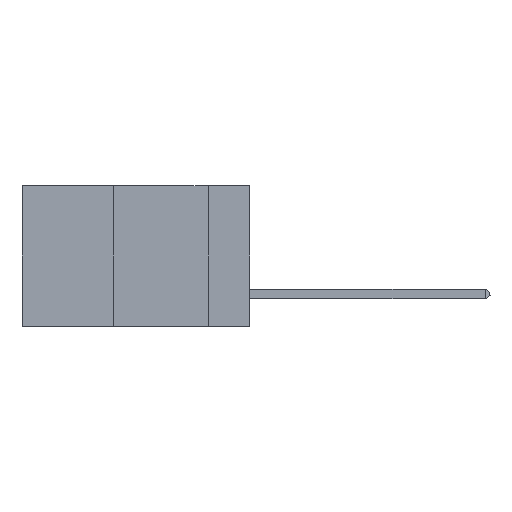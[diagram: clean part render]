
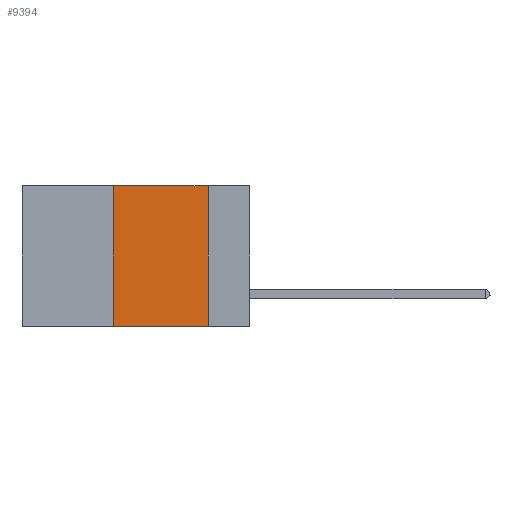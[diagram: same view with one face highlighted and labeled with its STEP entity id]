
A CAD part, left-side view. The second image highlights one B-rep face of the part: STEP entity #9394.
In plain terms, the highlighted planar face has unit normal (-1, 0, 0).
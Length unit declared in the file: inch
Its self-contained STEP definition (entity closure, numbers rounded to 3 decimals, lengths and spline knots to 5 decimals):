
#344 = VECTOR ( 'NONE', #7917, 39.37008 ) ;
#497 = DIRECTION ( 'NONE',  ( 0., 0., -1. ) ) ;
#654 = PLANE ( 'NONE',  #12254 ) ;
#928 = EDGE_CURVE ( 'NONE', #20056, #16907, #2650, .T. ) ;
#1216 = CARTESIAN_POINT ( 'NONE',  ( 0., 0.11, 0. ) ) ;
#1509 = DIRECTION ( 'NONE',  ( 0., -1., 0. ) ) ;
#1728 = EDGE_LOOP ( 'NONE', ( #21644, #12761, #12477, #19996 ) ) ;
#2590 = CARTESIAN_POINT ( 'NONE',  ( 0., 0.36, 0. ) ) ;
#2650 = LINE ( 'NONE', #2590, #22590 ) ;
#3061 = DIRECTION ( 'NONE',  ( 0., -1., 0. ) ) ;
#5105 = EDGE_CURVE ( 'NONE', #16907, #8506, #8698, .T. ) ;
#5330 = EDGE_CURVE ( 'NONE', #20056, #7472, #7218, .T. ) ;
#6297 = VECTOR ( 'NONE', #3061, 39.37008 ) ;
#6865 = CARTESIAN_POINT ( 'NONE',  ( 0., 0.36, -0.37 ) ) ;
#7218 = LINE ( 'NONE', #16076, #6297 ) ;
#7472 = VERTEX_POINT ( 'NONE', #23573 ) ;
#7917 = DIRECTION ( 'NONE',  ( 0., 0., -1. ) ) ;
#8506 = VERTEX_POINT ( 'NONE', #1216 ) ;
#8698 = LINE ( 'NONE', #10335, #10439 ) ;
#9394 = ADVANCED_FACE ( 'NONE', ( #14055 ), #654, .F. ) ;
#9648 = CARTESIAN_POINT ( 'NONE',  ( 0., 0.11, 0. ) ) ;
#10335 = CARTESIAN_POINT ( 'NONE',  ( 0., 0.6, 0. ) ) ;
#10439 = VECTOR ( 'NONE', #1509, 39.37008 ) ;
#10499 = CARTESIAN_POINT ( 'NONE',  ( 0., 0.36, 0. ) ) ;
#11791 = DIRECTION ( 'NONE',  ( 1., 0., 0. ) ) ;
#12254 = AXIS2_PLACEMENT_3D ( 'NONE', #17442, #11791, #497 ) ;
#12477 = ORIENTED_EDGE ( 'NONE', *, *, #928, .F. ) ;
#12761 = ORIENTED_EDGE ( 'NONE', *, *, #5105, .F. ) ;
#13874 = DIRECTION ( 'NONE',  ( 0., 0., 1. ) ) ;
#14055 = FACE_OUTER_BOUND ( 'NONE', #1728, .T. ) ;
#16010 = EDGE_CURVE ( 'NONE', #8506, #7472, #16502, .T. ) ;
#16076 = CARTESIAN_POINT ( 'NONE',  ( 0., 0.6, -0.37 ) ) ;
#16502 = LINE ( 'NONE', #9648, #344 ) ;
#16907 = VERTEX_POINT ( 'NONE', #10499 ) ;
#17442 = CARTESIAN_POINT ( 'NONE',  ( 0., 0.6, 0. ) ) ;
#19996 = ORIENTED_EDGE ( 'NONE', *, *, #5330, .T. ) ;
#20056 = VERTEX_POINT ( 'NONE', #6865 ) ;
#21644 = ORIENTED_EDGE ( 'NONE', *, *, #16010, .F. ) ;
#22590 = VECTOR ( 'NONE', #13874, 39.37008 ) ;
#23573 = CARTESIAN_POINT ( 'NONE',  ( 0., 0.11, -0.37 ) ) ;
